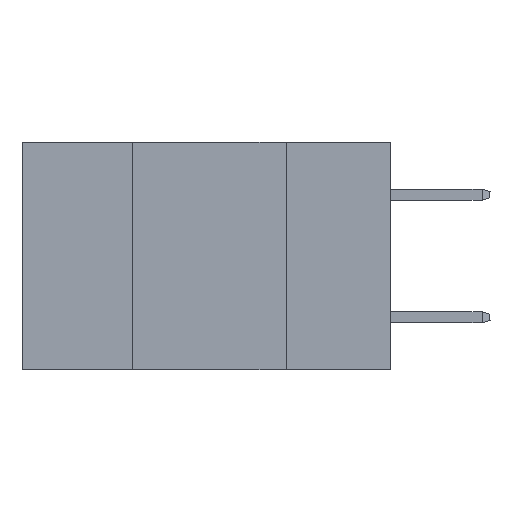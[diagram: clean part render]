
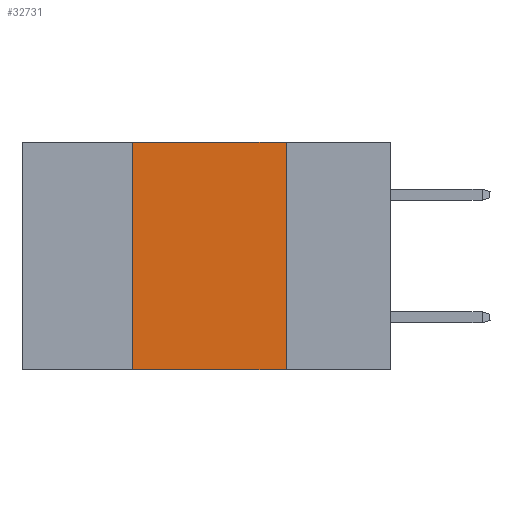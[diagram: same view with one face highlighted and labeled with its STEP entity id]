
A CAD part, left-side view. The second image highlights one B-rep face of the part: STEP entity #32731.
In plain terms, the highlighted planar face has unit normal (-1, 0, 0).
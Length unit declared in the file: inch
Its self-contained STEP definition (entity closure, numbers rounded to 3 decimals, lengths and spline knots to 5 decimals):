
#798 = VERTEX_POINT ( 'NONE', #36236 ) ;
#1336 = LINE ( 'NONE', #11459, #32527 ) ;
#2000 = EDGE_CURVE ( 'NONE', #15077, #38343, #1336, .T. ) ;
#2075 = CARTESIAN_POINT ( 'NONE',  ( 0., 0.6, -0.37 ) ) ;
#3165 = LINE ( 'NONE', #32573, #18333 ) ;
#3389 = FACE_OUTER_BOUND ( 'NONE', #29831, .T. ) ;
#5123 = DIRECTION ( 'NONE',  ( 0., -1., 0. ) ) ;
#6142 = ORIENTED_EDGE ( 'NONE', *, *, #14648, .T. ) ;
#7657 = CARTESIAN_POINT ( 'NONE',  ( 0., 0.42, -0.37 ) ) ;
#9768 = EDGE_CURVE ( 'NONE', #798, #15077, #11181, .T. ) ;
#10282 = CARTESIAN_POINT ( 'NONE',  ( 0., 0.6, 0. ) ) ;
#11181 = LINE ( 'NONE', #28615, #24387 ) ;
#11459 = CARTESIAN_POINT ( 'NONE',  ( 0., 0.17, 0. ) ) ;
#13337 = DIRECTION ( 'NONE',  ( 1., 0., 0. ) ) ;
#13581 = DIRECTION ( 'NONE',  ( 0., -1., 0. ) ) ;
#14000 = ORIENTED_EDGE ( 'NONE', *, *, #9768, .F. ) ;
#14503 = DIRECTION ( 'NONE',  ( 0., 0., 1. ) ) ;
#14648 = EDGE_CURVE ( 'NONE', #34310, #38343, #32230, .T. ) ;
#15077 = VERTEX_POINT ( 'NONE', #16069 ) ;
#16069 = CARTESIAN_POINT ( 'NONE',  ( 0., 0.17, 0. ) ) ;
#18333 = VECTOR ( 'NONE', #14503, 39.37008 ) ;
#20123 = ORIENTED_EDGE ( 'NONE', *, *, #2000, .F. ) ;
#20531 = DIRECTION ( 'NONE',  ( 0., 0., -1. ) ) ;
#23239 = VECTOR ( 'NONE', #5123, 39.37008 ) ;
#24387 = VECTOR ( 'NONE', #13581, 39.37008 ) ;
#28354 = PLANE ( 'NONE',  #37027 ) ;
#28615 = CARTESIAN_POINT ( 'NONE',  ( 0., 0.6, 0. ) ) ;
#29243 = CARTESIAN_POINT ( 'NONE',  ( 0., 0.17, -0.37 ) ) ;
#29831 = EDGE_LOOP ( 'NONE', ( #20123, #14000, #30064, #6142 ) ) ;
#30064 = ORIENTED_EDGE ( 'NONE', *, *, #37754, .F. ) ;
#32230 = LINE ( 'NONE', #2075, #23239 ) ;
#32527 = VECTOR ( 'NONE', #20531, 39.37008 ) ;
#32573 = CARTESIAN_POINT ( 'NONE',  ( 0., 0.42, 0. ) ) ;
#32731 = ADVANCED_FACE ( 'NONE', ( #3389 ), #28354, .F. ) ;
#34310 = VERTEX_POINT ( 'NONE', #7657 ) ;
#34381 = DIRECTION ( 'NONE',  ( 0., 0., -1. ) ) ;
#36236 = CARTESIAN_POINT ( 'NONE',  ( 0., 0.42, 0. ) ) ;
#37027 = AXIS2_PLACEMENT_3D ( 'NONE', #10282, #13337, #34381 ) ;
#37754 = EDGE_CURVE ( 'NONE', #34310, #798, #3165, .T. ) ;
#38343 = VERTEX_POINT ( 'NONE', #29243 ) ;
